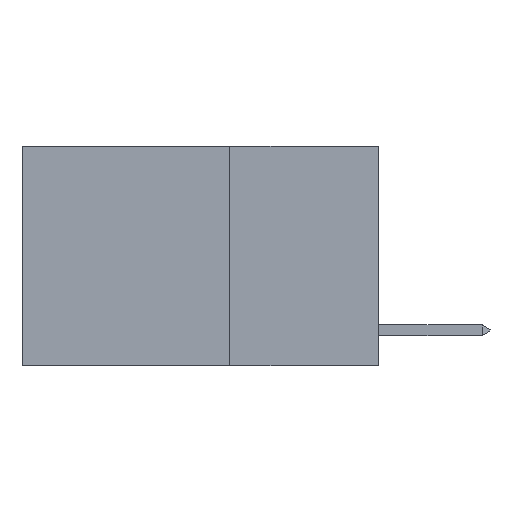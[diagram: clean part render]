
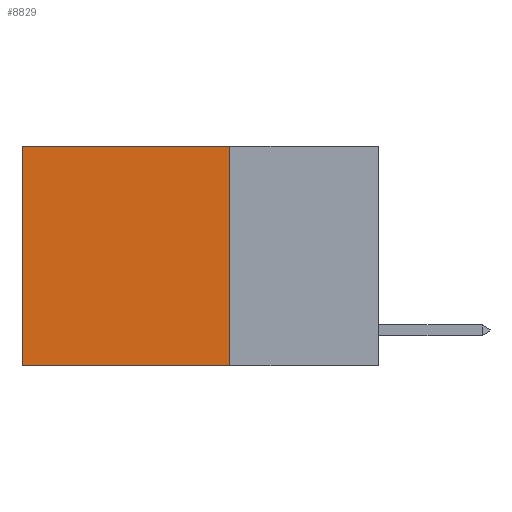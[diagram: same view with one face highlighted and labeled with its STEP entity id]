
A CAD part, left-side view. The second image highlights one B-rep face of the part: STEP entity #8829.
In plain terms, the highlighted planar face has unit normal (-1, 0, 0).
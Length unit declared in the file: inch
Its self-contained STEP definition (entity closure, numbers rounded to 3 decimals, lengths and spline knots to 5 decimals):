
#60 = CARTESIAN_POINT ( 'NONE',  ( 0.2625, 0.25, 0. ) ) ;
#1294 = CARTESIAN_POINT ( 'NONE',  ( 0.2625, 0.25, 0. ) ) ;
#1710 = CARTESIAN_POINT ( 'NONE',  ( 0.2625, 0.6, 0. ) ) ;
#2057 = CARTESIAN_POINT ( 'NONE',  ( 0.2625, 0.6, 0. ) ) ;
#2798 = PLANE ( 'NONE',  #7491 ) ;
#3469 = EDGE_CURVE ( 'NONE', #5135, #3475, #9770, .T. ) ;
#3475 = VERTEX_POINT ( 'NONE', #2057 ) ;
#3780 = LINE ( 'NONE', #60, #11453 ) ;
#3929 = EDGE_CURVE ( 'NONE', #3475, #6275, #15596, .T. ) ;
#4003 = EDGE_LOOP ( 'NONE', ( #6427, #7628, #9105, #11382 ) ) ;
#4130 = DIRECTION ( 'NONE',  ( 1., 0., 0. ) ) ;
#4447 = DIRECTION ( 'NONE',  ( 0., 0., -1. ) ) ;
#5135 = VERTEX_POINT ( 'NONE', #11272 ) ;
#6194 = CARTESIAN_POINT ( 'NONE',  ( 0.2625, 0.25, 0. ) ) ;
#6216 = VECTOR ( 'NONE', #15543, 39.37008 ) ;
#6275 = VERTEX_POINT ( 'NONE', #15708 ) ;
#6304 = DIRECTION ( 'NONE',  ( 0., 1., 0. ) ) ;
#6427 = ORIENTED_EDGE ( 'NONE', *, *, #3929, .T. ) ;
#6539 = FACE_OUTER_BOUND ( 'NONE', #4003, .T. ) ;
#7035 = DIRECTION ( 'NONE',  ( 0., 0., -1. ) ) ;
#7491 = AXIS2_PLACEMENT_3D ( 'NONE', #1294, #4130, #13568 ) ;
#7628 = ORIENTED_EDGE ( 'NONE', *, *, #13794, .F. ) ;
#8829 = ADVANCED_FACE ( 'NONE', ( #6539 ), #2798, .F. ) ;
#9105 = ORIENTED_EDGE ( 'NONE', *, *, #15996, .F. ) ;
#9770 = LINE ( 'NONE', #6194, #6216 ) ;
#10684 = VERTEX_POINT ( 'NONE', #16403 ) ;
#11272 = CARTESIAN_POINT ( 'NONE',  ( 0.2625, 0.25, 0. ) ) ;
#11382 = ORIENTED_EDGE ( 'NONE', *, *, #3469, .T. ) ;
#11453 = VECTOR ( 'NONE', #7035, 39.37008 ) ;
#12493 = VECTOR ( 'NONE', #4447, 39.37008 ) ;
#13568 = DIRECTION ( 'NONE',  ( 0., 0., -1. ) ) ;
#13794 = EDGE_CURVE ( 'NONE', #10684, #6275, #16758, .T. ) ;
#14317 = CARTESIAN_POINT ( 'NONE',  ( 0.2625, 0.25, -0.37 ) ) ;
#15543 = DIRECTION ( 'NONE',  ( 0., 1., 0. ) ) ;
#15596 = LINE ( 'NONE', #1710, #12493 ) ;
#15708 = CARTESIAN_POINT ( 'NONE',  ( 0.2625, 0.6, -0.37 ) ) ;
#15996 = EDGE_CURVE ( 'NONE', #5135, #10684, #3780, .T. ) ;
#16403 = CARTESIAN_POINT ( 'NONE',  ( 0.2625, 0.25, -0.37 ) ) ;
#16758 = LINE ( 'NONE', #14317, #17147 ) ;
#17147 = VECTOR ( 'NONE', #6304, 39.37008 ) ;
